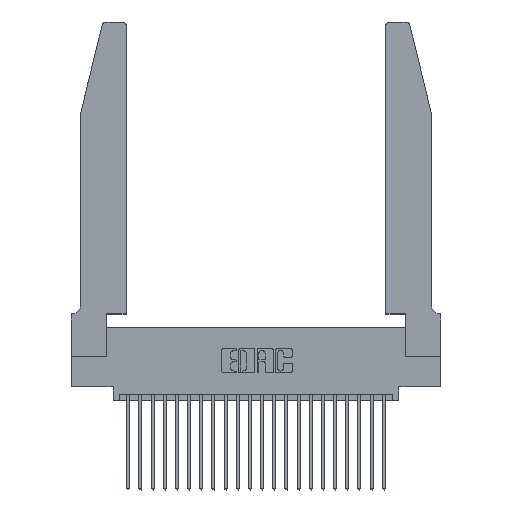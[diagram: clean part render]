
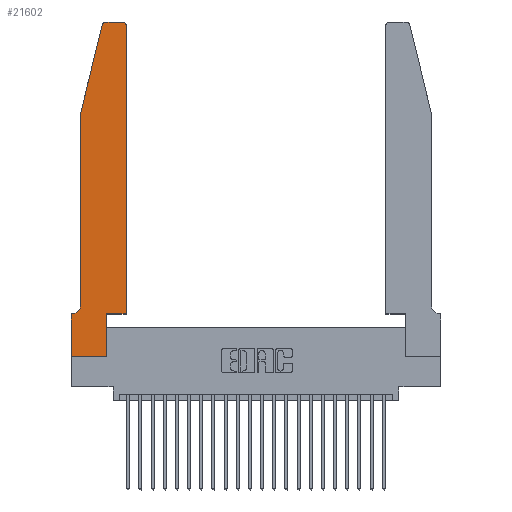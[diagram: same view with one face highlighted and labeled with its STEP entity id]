
A CAD part, top view. The second image highlights one B-rep face of the part: STEP entity #21602.
In plain terms, the highlighted planar face has unit normal (0, 0, 1).
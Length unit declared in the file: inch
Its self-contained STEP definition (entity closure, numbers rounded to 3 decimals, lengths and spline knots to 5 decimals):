
#213 = DIRECTION ( 'NONE',  ( 0., -1., 0. ) ) ;
#216 = CARTESIAN_POINT ( 'NONE',  ( 0.4505, 0.35, 0.37 ) ) ;
#300 = CARTESIAN_POINT ( 'NONE',  ( 0.2865, 0., 0.37 ) ) ;
#515 = VERTEX_POINT ( 'NONE', #13361 ) ;
#857 = LINE ( 'NONE', #23274, #10716 ) ;
#872 = DIRECTION ( 'NONE',  ( 0., 0., 1. ) ) ;
#898 = ORIENTED_EDGE ( 'NONE', *, *, #4601, .T. ) ;
#1050 = CIRCLE ( 'NONE', #24408, 0.03 ) ;
#1442 = CARTESIAN_POINT ( 'NONE',  ( 0.0755, 2., 0.37 ) ) ;
#1716 = VERTEX_POINT ( 'NONE', #24654 ) ;
#1873 = ORIENTED_EDGE ( 'NONE', *, *, #23665, .T. ) ;
#1895 = VERTEX_POINT ( 'NONE', #7767 ) ;
#1960 = CIRCLE ( 'NONE', #4581, 0.03 ) ;
#2181 = VECTOR ( 'NONE', #2235, 39.37008 ) ;
#2209 = EDGE_LOOP ( 'NONE', ( #17829, #24652, #5251, #898, #5355, #2833, #6590, #14982, #22478, #1873, #9236, #15030 ) ) ;
#2235 = DIRECTION ( 'NONE',  ( 1., 0., 0. ) ) ;
#2833 = ORIENTED_EDGE ( 'NONE', *, *, #4356, .T. ) ;
#3751 = LINE ( 'NONE', #1442, #23518 ) ;
#3908 = EDGE_CURVE ( 'NONE', #11253, #515, #16208, .T. ) ;
#4040 = VERTEX_POINT ( 'NONE', #7935 ) ;
#4093 = VECTOR ( 'NONE', #24069, 39.37008 ) ;
#4356 = EDGE_CURVE ( 'NONE', #9049, #12976, #6461, .T. ) ;
#4387 = CARTESIAN_POINT ( 'NONE',  ( 0.0055, 0.42, 0.37 ) ) ;
#4581 = AXIS2_PLACEMENT_3D ( 'NONE', #20823, #9394, #22688 ) ;
#4601 = EDGE_CURVE ( 'NONE', #20845, #5103, #857, .T. ) ;
#5103 = VERTEX_POINT ( 'NONE', #9643 ) ;
#5207 = VECTOR ( 'NONE', #19894, 39.37008 ) ;
#5251 = ORIENTED_EDGE ( 'NONE', *, *, #21232, .T. ) ;
#5355 = ORIENTED_EDGE ( 'NONE', *, *, #7487, .T. ) ;
#6130 = CARTESIAN_POINT ( 'NONE',  ( 0.0755, 2., 0.37 ) ) ;
#6383 = DIRECTION ( 'NONE',  ( -1., 0., 0. ) ) ;
#6461 = LINE ( 'NONE', #7055, #7090 ) ;
#6590 = ORIENTED_EDGE ( 'NONE', *, *, #10327, .T. ) ;
#6803 = CARTESIAN_POINT ( 'NONE',  ( 0.2865, 0.35, 0.37 ) ) ;
#7055 = CARTESIAN_POINT ( 'NONE',  ( 0.0755, 0.35, 0.37 ) ) ;
#7090 = VECTOR ( 'NONE', #18568, 39.37008 ) ;
#7487 = EDGE_CURVE ( 'NONE', #5103, #9049, #15487, .T. ) ;
#7600 = DIRECTION ( 'NONE',  ( 0., 0., 1. ) ) ;
#7767 = CARTESIAN_POINT ( 'NONE',  ( 0.4505, 0.35, 0.37 ) ) ;
#7935 = CARTESIAN_POINT ( 'NONE',  ( 0.25487, 2.72718, 0.37 ) ) ;
#7988 = DIRECTION ( 'NONE',  ( 0., -1., 0. ) ) ;
#8731 = LINE ( 'NONE', #21321, #18952 ) ;
#9049 = VERTEX_POINT ( 'NONE', #24354 ) ;
#9236 = ORIENTED_EDGE ( 'NONE', *, *, #11989, .T. ) ;
#9394 = DIRECTION ( 'NONE',  ( 0., 0., 1. ) ) ;
#9643 = CARTESIAN_POINT ( 'NONE',  ( 0.0755, 0.42, 0.37 ) ) ;
#9957 = CARTESIAN_POINT ( 'NONE',  ( 0.4505, 2.72, 0.37 ) ) ;
#10327 = EDGE_CURVE ( 'NONE', #12976, #1716, #8731, .T. ) ;
#10716 = VECTOR ( 'NONE', #213, 39.37008 ) ;
#11253 = VERTEX_POINT ( 'NONE', #18276 ) ;
#11479 = CARTESIAN_POINT ( 'NONE',  ( 0.2605, 2.75, 0.37 ) ) ;
#11989 = EDGE_CURVE ( 'NONE', #1895, #19531, #19515, .T. ) ;
#12645 = PLANE ( 'NONE',  #21190 ) ;
#12976 = VERTEX_POINT ( 'NONE', #19461 ) ;
#13361 = CARTESIAN_POINT ( 'NONE',  ( 0.284, 2.75, 0.37 ) ) ;
#14634 = DIRECTION ( 'NONE',  ( 1., 0., 0. ) ) ;
#14675 = LINE ( 'NONE', #21956, #19046 ) ;
#14982 = ORIENTED_EDGE ( 'NONE', *, *, #22781, .T. ) ;
#15030 = ORIENTED_EDGE ( 'NONE', *, *, #20477, .T. ) ;
#15487 = CIRCLE ( 'NONE', #22554, 0.07 ) ;
#16208 = LINE ( 'NONE', #11479, #17380 ) ;
#16346 = DIRECTION ( 'NONE',  ( 0., 1., 0. ) ) ;
#17165 = EDGE_CURVE ( 'NONE', #23215, #17764, #14675, .T. ) ;
#17380 = VECTOR ( 'NONE', #22805, 39.37008 ) ;
#17764 = VERTEX_POINT ( 'NONE', #6803 ) ;
#17829 = ORIENTED_EDGE ( 'NONE', *, *, #3908, .T. ) ;
#17961 = DIRECTION ( 'NONE',  ( 0., 0., -1. ) ) ;
#18017 = CARTESIAN_POINT ( 'NONE',  ( 0., 0., 0.37 ) ) ;
#18276 = CARTESIAN_POINT ( 'NONE',  ( 0.4205, 2.75, 0.37 ) ) ;
#18568 = DIRECTION ( 'NONE',  ( -1., 0., 0. ) ) ;
#18952 = VECTOR ( 'NONE', #7988, 39.37008 ) ;
#19046 = VECTOR ( 'NONE', #16346, 39.37008 ) ;
#19078 = CARTESIAN_POINT ( 'NONE',  ( 0.284, 2.72, 0.37 ) ) ;
#19349 = EDGE_CURVE ( 'NONE', #515, #4040, #1050, .T. ) ;
#19395 = LINE ( 'NONE', #18017, #5207 ) ;
#19461 = CARTESIAN_POINT ( 'NONE',  ( 0., 0.35, 0.37 ) ) ;
#19515 = LINE ( 'NONE', #23989, #4093 ) ;
#19531 = VERTEX_POINT ( 'NONE', #9957 ) ;
#19894 = DIRECTION ( 'NONE',  ( 1., 0., 0. ) ) ;
#20316 = FACE_OUTER_BOUND ( 'NONE', #2209, .T. ) ;
#20477 = EDGE_CURVE ( 'NONE', #19531, #11253, #1960, .T. ) ;
#20615 = DIRECTION ( 'NONE',  ( -0.239, -0.971, 0. ) ) ;
#20823 = CARTESIAN_POINT ( 'NONE',  ( 0.4205, 2.72, 0.37 ) ) ;
#20845 = VERTEX_POINT ( 'NONE', #6130 ) ;
#20961 = DIRECTION ( 'NONE',  ( 1., 0., 0. ) ) ;
#21190 = AXIS2_PLACEMENT_3D ( 'NONE', #23653, #872, #14634 ) ;
#21232 = EDGE_CURVE ( 'NONE', #4040, #20845, #3751, .T. ) ;
#21321 = CARTESIAN_POINT ( 'NONE',  ( 0., 0., 0.37 ) ) ;
#21602 = ADVANCED_FACE ( 'NONE', ( #20316 ), #12645, .T. ) ;
#21956 = CARTESIAN_POINT ( 'NONE',  ( 0.2865, 0.35, 0.37 ) ) ;
#22478 = ORIENTED_EDGE ( 'NONE', *, *, #17165, .T. ) ;
#22554 = AXIS2_PLACEMENT_3D ( 'NONE', #4387, #17961, #6383 ) ;
#22603 = LINE ( 'NONE', #216, #2181 ) ;
#22688 = DIRECTION ( 'NONE',  ( 1., 0., 0. ) ) ;
#22781 = EDGE_CURVE ( 'NONE', #1716, #23215, #19395, .T. ) ;
#22805 = DIRECTION ( 'NONE',  ( -1., 0., 0. ) ) ;
#23215 = VERTEX_POINT ( 'NONE', #300 ) ;
#23274 = CARTESIAN_POINT ( 'NONE',  ( 0.0755, 2., 0.37 ) ) ;
#23518 = VECTOR ( 'NONE', #20615, 39.37008 ) ;
#23653 = CARTESIAN_POINT ( 'NONE',  ( 0., 0.35, 0.37 ) ) ;
#23665 = EDGE_CURVE ( 'NONE', #17764, #1895, #22603, .T. ) ;
#23989 = CARTESIAN_POINT ( 'NONE',  ( 0.4505, 0.35, 0.37 ) ) ;
#24069 = DIRECTION ( 'NONE',  ( 0., 1., 0. ) ) ;
#24354 = CARTESIAN_POINT ( 'NONE',  ( 0.0055, 0.35, 0.37 ) ) ;
#24408 = AXIS2_PLACEMENT_3D ( 'NONE', #19078, #7600, #20961 ) ;
#24652 = ORIENTED_EDGE ( 'NONE', *, *, #19349, .T. ) ;
#24654 = CARTESIAN_POINT ( 'NONE',  ( 0., 0., 0.37 ) ) ;
